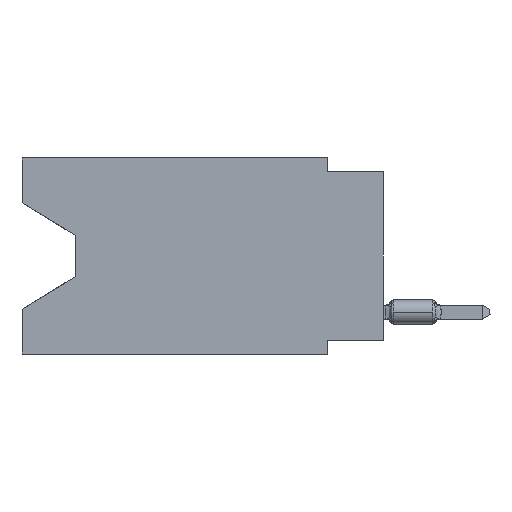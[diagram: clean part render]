
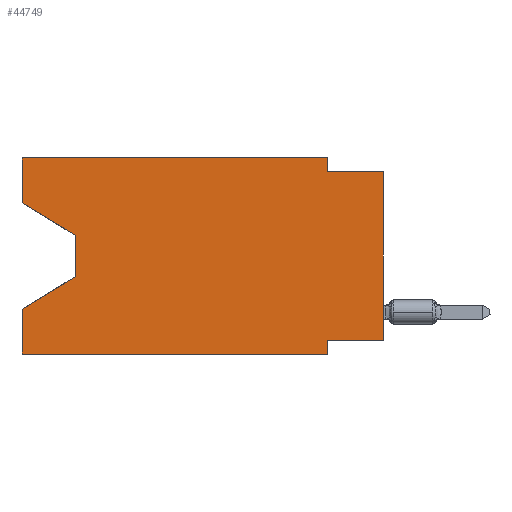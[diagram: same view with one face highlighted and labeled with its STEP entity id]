
A CAD part, left-side view. The second image highlights one B-rep face of the part: STEP entity #44749.
In plain terms, the highlighted planar face has unit normal (-1, 0, 0).
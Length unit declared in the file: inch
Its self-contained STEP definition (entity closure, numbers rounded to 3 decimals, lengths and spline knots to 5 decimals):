
#880 = CARTESIAN_POINT ( 'NONE',  ( 0., 0.645, -0.08025 ) ) ;
#1822 = CARTESIAN_POINT ( 'NONE',  ( 0., 0.645, 0. ) ) ;
#2346 = VECTOR ( 'NONE', #44924, 39.37008 ) ;
#3033 = VERTEX_POINT ( 'NONE', #27014 ) ;
#3073 = CARTESIAN_POINT ( 'NONE',  ( 0., 0., -0.025 ) ) ;
#4204 = VERTEX_POINT ( 'NONE', #50981 ) ;
#4524 = LINE ( 'NONE', #16158, #56650 ) ;
#4599 = DIRECTION ( 'NONE',  ( 0., 1., 0. ) ) ;
#5750 = ORIENTED_EDGE ( 'NONE', *, *, #56265, .T. ) ;
#6367 = LINE ( 'NONE', #880, #7053 ) ;
#6396 = VECTOR ( 'NONE', #4599, 39.37008 ) ;
#6460 = LINE ( 'NONE', #16734, #35448 ) ;
#6547 = VECTOR ( 'NONE', #25663, 39.37008 ) ;
#6963 = CARTESIAN_POINT ( 'NONE',  ( 0., 0.1, 0. ) ) ;
#7053 = VECTOR ( 'NONE', #26215, 39.37008 ) ;
#7271 = VERTEX_POINT ( 'NONE', #36627 ) ;
#9504 = VERTEX_POINT ( 'NONE', #24561 ) ;
#9976 = DIRECTION ( 'NONE',  ( 0., 0.855, -0.519 ) ) ;
#12488 = VERTEX_POINT ( 'NONE', #36912 ) ;
#12580 = EDGE_CURVE ( 'NONE', #55550, #15589, #6460, .T. ) ;
#13561 = EDGE_CURVE ( 'NONE', #4204, #7271, #64083, .T. ) ;
#15138 = ORIENTED_EDGE ( 'NONE', *, *, #65333, .T. ) ;
#15244 = EDGE_CURVE ( 'NONE', #39988, #3033, #30487, .T. ) ;
#15589 = VERTEX_POINT ( 'NONE', #3073 ) ;
#16158 = CARTESIAN_POINT ( 'NONE',  ( 0., 0.1, -0.35 ) ) ;
#16734 = CARTESIAN_POINT ( 'NONE',  ( 0., 0., 0. ) ) ;
#17238 = DIRECTION ( 'NONE',  ( 0., -1., 0. ) ) ;
#18120 = LINE ( 'NONE', #59815, #25135 ) ;
#20767 = VECTOR ( 'NONE', #42971, 39.37008 ) ;
#21372 = CARTESIAN_POINT ( 'NONE',  ( 0., 0., -0.325 ) ) ;
#21616 = ORIENTED_EDGE ( 'NONE', *, *, #29982, .F. ) ;
#21798 = ORIENTED_EDGE ( 'NONE', *, *, #15244, .T. ) ;
#22104 = LINE ( 'NONE', #58651, #20767 ) ;
#22289 = PLANE ( 'NONE',  #55871 ) ;
#22611 = DIRECTION ( 'NONE',  ( 1., 0., 0. ) ) ;
#22953 = CARTESIAN_POINT ( 'NONE',  ( 0., 0.645, 0. ) ) ;
#24001 = VECTOR ( 'NONE', #39072, 39.37008 ) ;
#24561 = CARTESIAN_POINT ( 'NONE',  ( 0., 0.1, -0.325 ) ) ;
#25135 = VECTOR ( 'NONE', #36202, 39.37008 ) ;
#25556 = CARTESIAN_POINT ( 'NONE',  ( 0., 0.645, -0.35 ) ) ;
#25663 = DIRECTION ( 'NONE',  ( 0., -1., 0. ) ) ;
#25683 = CARTESIAN_POINT ( 'NONE',  ( 0., 0., -0.325 ) ) ;
#26205 = ORIENTED_EDGE ( 'NONE', *, *, #55881, .F. ) ;
#26215 = DIRECTION ( 'NONE',  ( 0., -0.855, -0.519 ) ) ;
#26523 = CARTESIAN_POINT ( 'NONE',  ( 0., 0.1, -0.025 ) ) ;
#27014 = CARTESIAN_POINT ( 'NONE',  ( 0., 0.645, -0.26975 ) ) ;
#29124 = LINE ( 'NONE', #49999, #24001 ) ;
#29727 = VECTOR ( 'NONE', #64407, 39.37008 ) ;
#29855 = EDGE_LOOP ( 'NONE', ( #15138, #5750, #21798, #26205, #60611, #63471, #55498, #63587, #33491, #21616, #38032, #41668 ) ) ;
#29982 = EDGE_CURVE ( 'NONE', #7271, #63967, #53797, .T. ) ;
#30487 = LINE ( 'NONE', #35966, #34620 ) ;
#30592 = LINE ( 'NONE', #21372, #6396 ) ;
#31142 = EDGE_CURVE ( 'NONE', #63967, #15589, #49716, .T. ) ;
#32282 = VECTOR ( 'NONE', #17238, 39.37008 ) ;
#33491 = ORIENTED_EDGE ( 'NONE', *, *, #31142, .F. ) ;
#34620 = VECTOR ( 'NONE', #9976, 39.37008 ) ;
#35245 = LINE ( 'NONE', #35923, #6547 ) ;
#35448 = VECTOR ( 'NONE', #37603, 39.37008 ) ;
#35923 = CARTESIAN_POINT ( 'NONE',  ( 0., 0.645, -0.35 ) ) ;
#35966 = CARTESIAN_POINT ( 'NONE',  ( 0., 0.55, -0.212 ) ) ;
#36202 = DIRECTION ( 'NONE',  ( 0., 0., 1. ) ) ;
#36627 = CARTESIAN_POINT ( 'NONE',  ( 0., 0.1, 0. ) ) ;
#36912 = CARTESIAN_POINT ( 'NONE',  ( 0., 0.55, -0.138 ) ) ;
#37027 = DIRECTION ( 'NONE',  ( 0., 0., -1. ) ) ;
#37603 = DIRECTION ( 'NONE',  ( 0., 0., 1. ) ) ;
#37685 = DIRECTION ( 'NONE',  ( 0., 0., -1. ) ) ;
#38032 = ORIENTED_EDGE ( 'NONE', *, *, #13561, .F. ) ;
#38362 = FACE_OUTER_BOUND ( 'NONE', #29855, .T. ) ;
#39072 = DIRECTION ( 'NONE',  ( 0., 0., 1. ) ) ;
#39477 = EDGE_CURVE ( 'NONE', #55550, #9504, #30592, .T. ) ;
#39920 = EDGE_CURVE ( 'NONE', #9504, #52287, #4524, .T. ) ;
#39988 = VERTEX_POINT ( 'NONE', #48973 ) ;
#41149 = EDGE_CURVE ( 'NONE', #60615, #52287, #35245, .T. ) ;
#41668 = ORIENTED_EDGE ( 'NONE', *, *, #54199, .F. ) ;
#42971 = DIRECTION ( 'NONE',  ( 0., 0., -1. ) ) ;
#44229 = CARTESIAN_POINT ( 'NONE',  ( 0., 0.1, -0.35 ) ) ;
#44749 = ADVANCED_FACE ( 'NONE', ( #38362 ), #22289, .F. ) ;
#44924 = DIRECTION ( 'NONE',  ( 0., 0., -1. ) ) ;
#48973 = CARTESIAN_POINT ( 'NONE',  ( 0., 0.55, -0.212 ) ) ;
#49716 = LINE ( 'NONE', #54823, #29727 ) ;
#49999 = CARTESIAN_POINT ( 'NONE',  ( 0., 0.645, 0. ) ) ;
#50981 = CARTESIAN_POINT ( 'NONE',  ( 0., 0.645, 0. ) ) ;
#52287 = VERTEX_POINT ( 'NONE', #44229 ) ;
#53797 = LINE ( 'NONE', #6963, #2346 ) ;
#54199 = EDGE_CURVE ( 'NONE', #55793, #4204, #29124, .T. ) ;
#54823 = CARTESIAN_POINT ( 'NONE',  ( 0., 0., -0.025 ) ) ;
#55498 = ORIENTED_EDGE ( 'NONE', *, *, #39477, .F. ) ;
#55550 = VERTEX_POINT ( 'NONE', #25683 ) ;
#55793 = VERTEX_POINT ( 'NONE', #60163 ) ;
#55871 = AXIS2_PLACEMENT_3D ( 'NONE', #22953, #22611, #37685 ) ;
#55881 = EDGE_CURVE ( 'NONE', #60615, #3033, #18120, .T. ) ;
#56265 = EDGE_CURVE ( 'NONE', #12488, #39988, #22104, .T. ) ;
#56650 = VECTOR ( 'NONE', #37027, 39.37008 ) ;
#58651 = CARTESIAN_POINT ( 'NONE',  ( 0., 0.55, -0.138 ) ) ;
#59815 = CARTESIAN_POINT ( 'NONE',  ( 0., 0.645, 0. ) ) ;
#60163 = CARTESIAN_POINT ( 'NONE',  ( 0., 0.645, -0.08025 ) ) ;
#60611 = ORIENTED_EDGE ( 'NONE', *, *, #41149, .T. ) ;
#60615 = VERTEX_POINT ( 'NONE', #25556 ) ;
#63471 = ORIENTED_EDGE ( 'NONE', *, *, #39920, .F. ) ;
#63587 = ORIENTED_EDGE ( 'NONE', *, *, #12580, .T. ) ;
#63967 = VERTEX_POINT ( 'NONE', #26523 ) ;
#64083 = LINE ( 'NONE', #1822, #32282 ) ;
#64407 = DIRECTION ( 'NONE',  ( 0., -1., 0. ) ) ;
#65333 = EDGE_CURVE ( 'NONE', #55793, #12488, #6367, .T. ) ;
